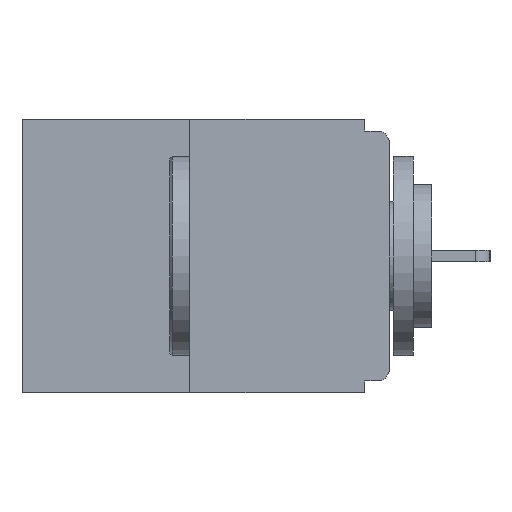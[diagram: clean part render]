
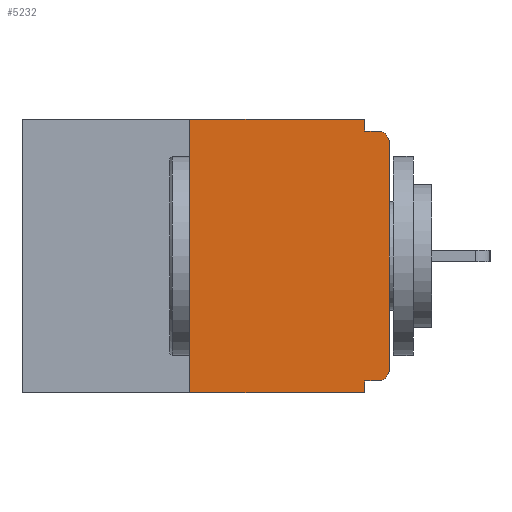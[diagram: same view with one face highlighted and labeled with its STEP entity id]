
A CAD part, left-side view. The second image highlights one B-rep face of the part: STEP entity #5232.
In plain terms, the highlighted planar face has unit normal (-1, 0, 0).
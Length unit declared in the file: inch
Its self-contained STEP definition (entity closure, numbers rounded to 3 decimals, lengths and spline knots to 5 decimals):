
#68 = CARTESIAN_POINT ( 'NONE',  ( 0., 0., -0.328 ) ) ;
#828 = DIRECTION ( 'NONE',  ( 0., 0., 1. ) ) ;
#1030 = LINE ( 'NONE', #18386, #12622 ) ;
#1311 = CARTESIAN_POINT ( 'NONE',  ( 0., 0.031, -0.343 ) ) ;
#1428 = CARTESIAN_POINT ( 'NONE',  ( 0., 0.031, 0. ) ) ;
#1489 = ORIENTED_EDGE ( 'NONE', *, *, #14477, .F. ) ;
#1857 = VERTEX_POINT ( 'NONE', #4224 ) ;
#1949 = DIRECTION ( 'NONE',  ( 0., 0., -1. ) ) ;
#2160 = CARTESIAN_POINT ( 'NONE',  ( 0., 0., -0.03 ) ) ;
#3021 = DIRECTION ( 'NONE',  ( -1., 0., 0. ) ) ;
#3177 = CARTESIAN_POINT ( 'NONE',  ( 0., 0.015, -0.313 ) ) ;
#3582 = EDGE_CURVE ( 'NONE', #3856, #3602, #12504, .T. ) ;
#3602 = VERTEX_POINT ( 'NONE', #12240 ) ;
#3680 = CARTESIAN_POINT ( 'NONE',  ( 0., 0.015, -0.03 ) ) ;
#3856 = VERTEX_POINT ( 'NONE', #27260 ) ;
#4224 = CARTESIAN_POINT ( 'NONE',  ( 0., 0.031, 0. ) ) ;
#4381 = ORIENTED_EDGE ( 'NONE', *, *, #22824, .F. ) ;
#4441 = VECTOR ( 'NONE', #16578, 39.37008 ) ;
#4865 = EDGE_CURVE ( 'NONE', #26014, #1857, #23542, .T. ) ;
#5232 = ADVANCED_FACE ( 'NONE', ( #15177 ), #23849, .F. ) ;
#5601 = ORIENTED_EDGE ( 'NONE', *, *, #4865, .F. ) ;
#5829 = LINE ( 'NONE', #1428, #8806 ) ;
#5937 = ORIENTED_EDGE ( 'NONE', *, *, #11070, .T. ) ;
#6109 = VECTOR ( 'NONE', #15272, 39.37008 ) ;
#6330 = VECTOR ( 'NONE', #27482, 39.37008 ) ;
#6359 = DIRECTION ( 'NONE',  ( 0., 1., 0. ) ) ;
#6635 = DIRECTION ( 'NONE',  ( 1., 0., 0. ) ) ;
#6979 = VECTOR ( 'NONE', #20647, 39.37008 ) ;
#7185 = CARTESIAN_POINT ( 'NONE',  ( 0., 0.25, -0.343 ) ) ;
#7216 = ORIENTED_EDGE ( 'NONE', *, *, #19036, .T. ) ;
#7489 = ORIENTED_EDGE ( 'NONE', *, *, #18916, .T. ) ;
#8123 = VERTEX_POINT ( 'NONE', #7185 ) ;
#8806 = VECTOR ( 'NONE', #18892, 39.37008 ) ;
#9530 = EDGE_CURVE ( 'NONE', #1857, #3856, #5829, .T. ) ;
#9765 = EDGE_CURVE ( 'NONE', #8123, #15992, #19245, .T. ) ;
#10456 = CARTESIAN_POINT ( 'NONE',  ( 0., 0.46, -0.343 ) ) ;
#10501 = VECTOR ( 'NONE', #828, 39.37008 ) ;
#11070 = EDGE_CURVE ( 'NONE', #16900, #20180, #12665, .T. ) ;
#11242 = VERTEX_POINT ( 'NONE', #2160 ) ;
#12018 = ORIENTED_EDGE ( 'NONE', *, *, #9530, .F. ) ;
#12225 = AXIS2_PLACEMENT_3D ( 'NONE', #3177, #3021, #26950 ) ;
#12240 = CARTESIAN_POINT ( 'NONE',  ( 0., 0.015, -0.015 ) ) ;
#12504 = LINE ( 'NONE', #16800, #6330 ) ;
#12622 = VECTOR ( 'NONE', #20531, 39.37008 ) ;
#12665 = CIRCLE ( 'NONE', #12225, 0.015 ) ;
#12720 = CARTESIAN_POINT ( 'NONE',  ( 0., 0.46, 0. ) ) ;
#13198 = CIRCLE ( 'NONE', #18198, 0.015 ) ;
#14477 = EDGE_CURVE ( 'NONE', #8123, #26014, #18646, .T. ) ;
#15177 = FACE_OUTER_BOUND ( 'NONE', #26798, .T. ) ;
#15272 = DIRECTION ( 'NONE',  ( 0., -1., 0. ) ) ;
#15992 = VERTEX_POINT ( 'NONE', #1311 ) ;
#16103 = CARTESIAN_POINT ( 'NONE',  ( 0., 0.25, 0. ) ) ;
#16400 = EDGE_CURVE ( 'NONE', #16900, #22897, #19573, .T. ) ;
#16504 = DIRECTION ( 'NONE',  ( 0., 0., -1. ) ) ;
#16578 = DIRECTION ( 'NONE',  ( 0., -1., 0. ) ) ;
#16800 = CARTESIAN_POINT ( 'NONE',  ( 0., 0., -0.015 ) ) ;
#16900 = VERTEX_POINT ( 'NONE', #18305 ) ;
#18198 = AXIS2_PLACEMENT_3D ( 'NONE', #3680, #23042, #16504 ) ;
#18305 = CARTESIAN_POINT ( 'NONE',  ( 0., 0.015, -0.328 ) ) ;
#18386 = CARTESIAN_POINT ( 'NONE',  ( 0., 0.031, -0.343 ) ) ;
#18646 = LINE ( 'NONE', #16103, #6979 ) ;
#18892 = DIRECTION ( 'NONE',  ( 0., 0., -1. ) ) ;
#18916 = EDGE_CURVE ( 'NONE', #20180, #11242, #24754, .T. ) ;
#19036 = EDGE_CURVE ( 'NONE', #11242, #3602, #13198, .T. ) ;
#19245 = LINE ( 'NONE', #10456, #6109 ) ;
#19573 = LINE ( 'NONE', #68, #23033 ) ;
#19925 = AXIS2_PLACEMENT_3D ( 'NONE', #21435, #6635, #1949 ) ;
#20180 = VERTEX_POINT ( 'NONE', #22604 ) ;
#20322 = CARTESIAN_POINT ( 'NONE',  ( 0., 0., 0. ) ) ;
#20531 = DIRECTION ( 'NONE',  ( 0., 0., -1. ) ) ;
#20647 = DIRECTION ( 'NONE',  ( 0., 0., 1. ) ) ;
#21435 = CARTESIAN_POINT ( 'NONE',  ( 0., 0.46, 0. ) ) ;
#22604 = CARTESIAN_POINT ( 'NONE',  ( 0., 0., -0.313 ) ) ;
#22784 = ORIENTED_EDGE ( 'NONE', *, *, #3582, .F. ) ;
#22824 = EDGE_CURVE ( 'NONE', #22897, #15992, #1030, .T. ) ;
#22897 = VERTEX_POINT ( 'NONE', #23660 ) ;
#23033 = VECTOR ( 'NONE', #6359, 39.37008 ) ;
#23042 = DIRECTION ( 'NONE',  ( -1., 0., 0. ) ) ;
#23542 = LINE ( 'NONE', #12720, #4441 ) ;
#23660 = CARTESIAN_POINT ( 'NONE',  ( 0., 0.031, -0.328 ) ) ;
#23849 = PLANE ( 'NONE',  #19925 ) ;
#24754 = LINE ( 'NONE', #20322, #10501 ) ;
#25075 = ORIENTED_EDGE ( 'NONE', *, *, #16400, .F. ) ;
#25342 = CARTESIAN_POINT ( 'NONE',  ( 0., 0.25, 0. ) ) ;
#26014 = VERTEX_POINT ( 'NONE', #25342 ) ;
#26798 = EDGE_LOOP ( 'NONE', ( #5601, #1489, #27133, #4381, #25075, #5937, #7489, #7216, #22784, #12018 ) ) ;
#26950 = DIRECTION ( 'NONE',  ( 0., 0., -1. ) ) ;
#27133 = ORIENTED_EDGE ( 'NONE', *, *, #9765, .T. ) ;
#27260 = CARTESIAN_POINT ( 'NONE',  ( 0., 0.031, -0.015 ) ) ;
#27482 = DIRECTION ( 'NONE',  ( 0., -1., 0. ) ) ;
